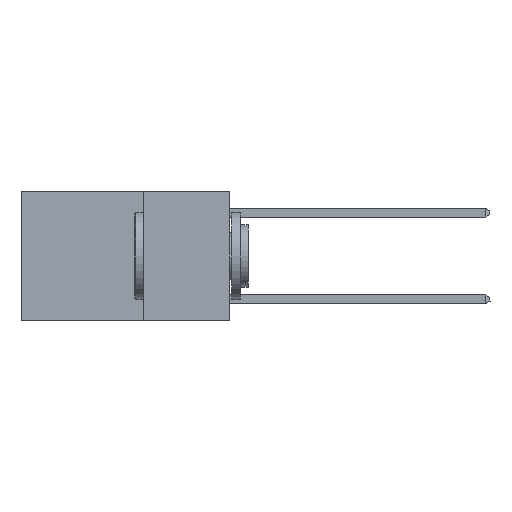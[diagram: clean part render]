
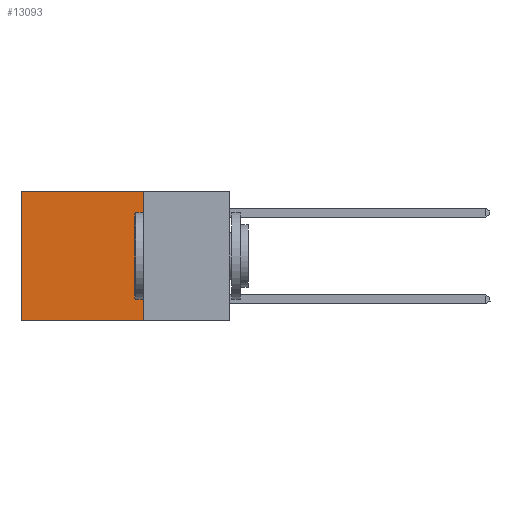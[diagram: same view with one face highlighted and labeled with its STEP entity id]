
A CAD part, left-side view. The second image highlights one B-rep face of the part: STEP entity #13093.
In plain terms, the highlighted planar face has unit normal (-1, 0, 0).
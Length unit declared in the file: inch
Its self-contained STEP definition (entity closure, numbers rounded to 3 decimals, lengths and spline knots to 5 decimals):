
#834 = CARTESIAN_POINT ( 'NONE',  ( 0.2625, 0.25, 0. ) ) ;
#1881 = EDGE_CURVE ( 'NONE', #21401, #13678, #28497, .T. ) ;
#2247 = VERTEX_POINT ( 'NONE', #23955 ) ;
#5409 = DIRECTION ( 'NONE',  ( 0., 0., -1. ) ) ;
#5447 = DIRECTION ( 'NONE',  ( 0., 0., -1. ) ) ;
#7524 = CARTESIAN_POINT ( 'NONE',  ( 0.2625, 0.25, -0.37 ) ) ;
#10055 = DIRECTION ( 'NONE',  ( 0., 1., 0. ) ) ;
#10521 = VERTEX_POINT ( 'NONE', #27813 ) ;
#12096 = PLANE ( 'NONE',  #27432 ) ;
#12220 = EDGE_LOOP ( 'NONE', ( #18973, #25159, #28444, #13631 ) ) ;
#13093 = ADVANCED_FACE ( 'NONE', ( #27283 ), #12096, .F. ) ;
#13516 = EDGE_CURVE ( 'NONE', #10521, #21401, #23071, .T. ) ;
#13631 = ORIENTED_EDGE ( 'NONE', *, *, #13516, .T. ) ;
#13678 = VERTEX_POINT ( 'NONE', #24289 ) ;
#14272 = CARTESIAN_POINT ( 'NONE',  ( 0.2625, 0.6, 0. ) ) ;
#14407 = CARTESIAN_POINT ( 'NONE',  ( 0.2625, 0.25, 0. ) ) ;
#17969 = VECTOR ( 'NONE', #22778, 39.37008 ) ;
#18824 = DIRECTION ( 'NONE',  ( 0., 1., 0. ) ) ;
#18973 = ORIENTED_EDGE ( 'NONE', *, *, #1881, .T. ) ;
#19784 = LINE ( 'NONE', #7524, #23992 ) ;
#21401 = VERTEX_POINT ( 'NONE', #14272 ) ;
#22778 = DIRECTION ( 'NONE',  ( 0., 0., -1. ) ) ;
#22987 = CARTESIAN_POINT ( 'NONE',  ( 0.2625, 0.6, 0. ) ) ;
#23071 = LINE ( 'NONE', #25384, #29010 ) ;
#23955 = CARTESIAN_POINT ( 'NONE',  ( 0.2625, 0.25, -0.37 ) ) ;
#23992 = VECTOR ( 'NONE', #10055, 39.37008 ) ;
#24067 = VECTOR ( 'NONE', #5447, 39.37008 ) ;
#24289 = CARTESIAN_POINT ( 'NONE',  ( 0.2625, 0.6, -0.37 ) ) ;
#25159 = ORIENTED_EDGE ( 'NONE', *, *, #28193, .F. ) ;
#25384 = CARTESIAN_POINT ( 'NONE',  ( 0.2625, 0.25, 0. ) ) ;
#26516 = LINE ( 'NONE', #14407, #24067 ) ;
#27283 = FACE_OUTER_BOUND ( 'NONE', #12220, .T. ) ;
#27432 = AXIS2_PLACEMENT_3D ( 'NONE', #834, #27922, #5409 ) ;
#27813 = CARTESIAN_POINT ( 'NONE',  ( 0.2625, 0.25, 0. ) ) ;
#27922 = DIRECTION ( 'NONE',  ( 1., 0., 0. ) ) ;
#28193 = EDGE_CURVE ( 'NONE', #2247, #13678, #19784, .T. ) ;
#28444 = ORIENTED_EDGE ( 'NONE', *, *, #28581, .F. ) ;
#28497 = LINE ( 'NONE', #22987, #17969 ) ;
#28581 = EDGE_CURVE ( 'NONE', #10521, #2247, #26516, .T. ) ;
#29010 = VECTOR ( 'NONE', #18824, 39.37008 ) ;
